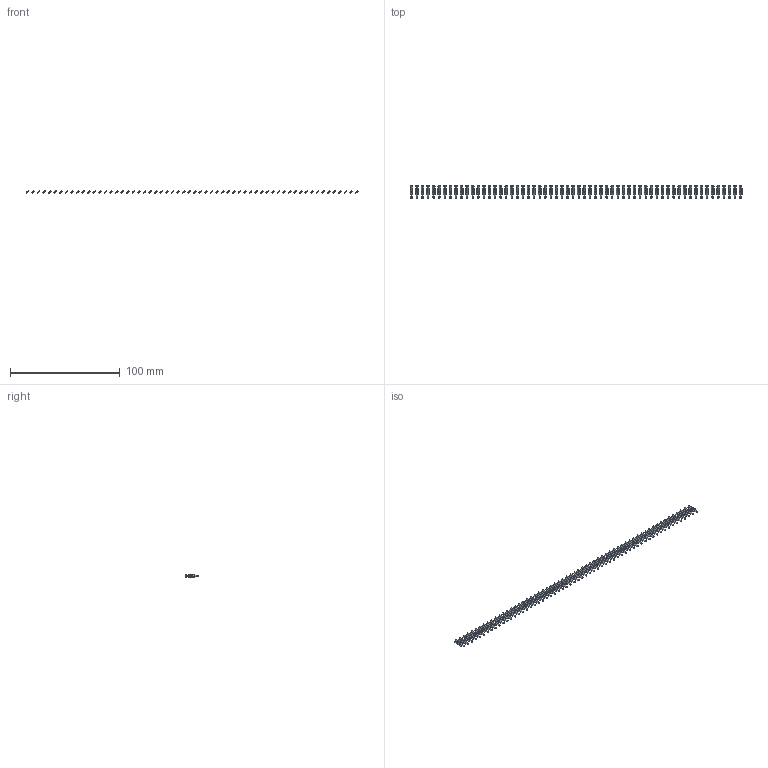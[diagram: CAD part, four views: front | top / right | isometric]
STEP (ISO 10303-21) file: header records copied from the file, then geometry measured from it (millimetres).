
FILE_DESCRIPTION (( 'STEP AP203' ), '1' );
FILE_NAME ('106-060-250-200.STEP', '2020-04-16T20:48:43', ( '' ), ( '' ), 'SwSTEP 2.0', 'SolidWorks 2016', '' );
FILE_SCHEMA (( 'CONFIG_CONTROL_DESIGN' ));
Length unit declared in the file: inch
Products named in the file (2): 106-060-250-200; 100-290-001_100-290-250
Assembly tree (60 placements, depth 2):
  106-060-250-200
    100-290-001_100-290-250  x60
Bounding box: 302.25 x 11.48 x 2.53 mm (x, y, z)
Volume: 936.3 mm3; surface area: 4401 mm2
Topology: 60 solids, 60 shells, 1440 faces, 3960 edges, 2640 vertices
Faces by surface type: plane 1200, cylinder 240
Entity records: 2846 total; most frequent: DIRECTION 244, CARTESIAN_POINT 209, ORIENTED_EDGE 132, CALENDAR_DATE 130, LOCAL_TIME 130, COORDINATED_UNIVERSAL_TIME_OFFSET 130, DATE_AND_TIME 130, AXIS2_PLACEMENT_3D 95
